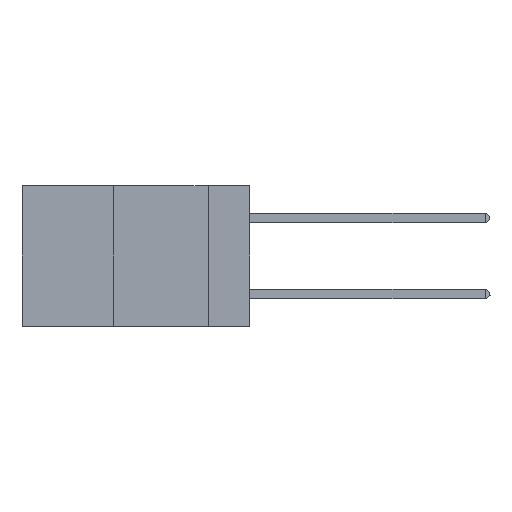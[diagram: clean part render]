
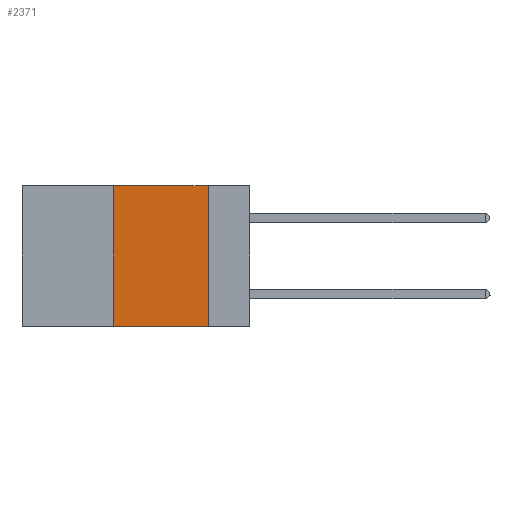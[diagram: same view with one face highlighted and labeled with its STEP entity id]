
A CAD part, left-side view. The second image highlights one B-rep face of the part: STEP entity #2371.
In plain terms, the highlighted planar face has unit normal (-1, 0, 0).
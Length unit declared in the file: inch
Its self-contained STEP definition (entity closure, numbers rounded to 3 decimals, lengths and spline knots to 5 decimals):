
#145 = VERTEX_POINT ( 'NONE', #5593 ) ;
#306 = EDGE_LOOP ( 'NONE', ( #5729, #7895, #6962, #683 ) ) ;
#460 = DIRECTION ( 'NONE',  ( 0., -1., 0. ) ) ;
#516 = CARTESIAN_POINT ( 'NONE',  ( 0., 0.6, 0. ) ) ;
#540 = VECTOR ( 'NONE', #460, 39.37008 ) ;
#683 = ORIENTED_EDGE ( 'NONE', *, *, #2261, .T. ) ;
#748 = DIRECTION ( 'NONE',  ( 0., 0., -1. ) ) ;
#751 = DIRECTION ( 'NONE',  ( 0., 0., 1. ) ) ;
#788 = CARTESIAN_POINT ( 'NONE',  ( 0., 0.36, 0. ) ) ;
#1796 = VECTOR ( 'NONE', #4539, 39.37008 ) ;
#2204 = CARTESIAN_POINT ( 'NONE',  ( 0., 0.36, -0.37 ) ) ;
#2261 = EDGE_CURVE ( 'NONE', #3599, #145, #5348, .T. ) ;
#2310 = FACE_OUTER_BOUND ( 'NONE', #306, .T. ) ;
#2371 = ADVANCED_FACE ( 'NONE', ( #2310 ), #7501, .F. ) ;
#2498 = VERTEX_POINT ( 'NONE', #7867 ) ;
#3035 = VERTEX_POINT ( 'NONE', #6886 ) ;
#3599 = VERTEX_POINT ( 'NONE', #2204 ) ;
#4539 = DIRECTION ( 'NONE',  ( 0., 0., -1. ) ) ;
#5150 = VECTOR ( 'NONE', #8135, 39.37008 ) ;
#5333 = LINE ( 'NONE', #516, #5150 ) ;
#5348 = LINE ( 'NONE', #5662, #540 ) ;
#5544 = EDGE_CURVE ( 'NONE', #3035, #2498, #5333, .T. ) ;
#5593 = CARTESIAN_POINT ( 'NONE',  ( 0., 0.11, -0.37 ) ) ;
#5662 = CARTESIAN_POINT ( 'NONE',  ( 0., 0.6, -0.37 ) ) ;
#5729 = ORIENTED_EDGE ( 'NONE', *, *, #7084, .F. ) ;
#6886 = CARTESIAN_POINT ( 'NONE',  ( 0., 0.36, 0. ) ) ;
#6947 = EDGE_CURVE ( 'NONE', #3599, #3035, #10800, .T. ) ;
#6962 = ORIENTED_EDGE ( 'NONE', *, *, #6947, .F. ) ;
#7084 = EDGE_CURVE ( 'NONE', #2498, #145, #8808, .T. ) ;
#7501 = PLANE ( 'NONE',  #9831 ) ;
#7867 = CARTESIAN_POINT ( 'NONE',  ( 0., 0.11, 0. ) ) ;
#7895 = ORIENTED_EDGE ( 'NONE', *, *, #5544, .F. ) ;
#8135 = DIRECTION ( 'NONE',  ( 0., -1., 0. ) ) ;
#8723 = CARTESIAN_POINT ( 'NONE',  ( 0., 0.11, 0. ) ) ;
#8808 = LINE ( 'NONE', #8723, #1796 ) ;
#9201 = CARTESIAN_POINT ( 'NONE',  ( 0., 0.6, 0. ) ) ;
#9343 = VECTOR ( 'NONE', #751, 39.37008 ) ;
#9831 = AXIS2_PLACEMENT_3D ( 'NONE', #9201, #10908, #748 ) ;
#10800 = LINE ( 'NONE', #788, #9343 ) ;
#10908 = DIRECTION ( 'NONE',  ( 1., 0., 0. ) ) ;
